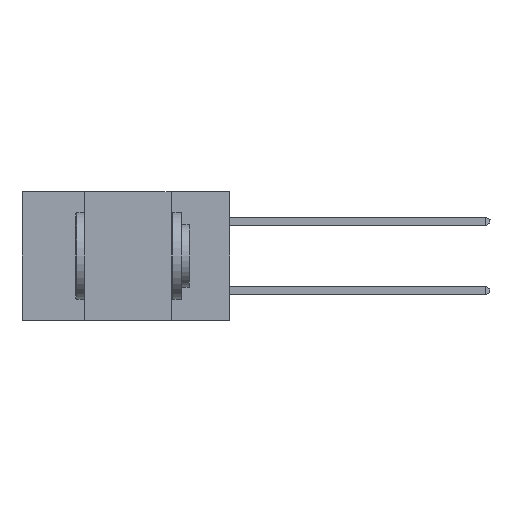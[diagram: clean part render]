
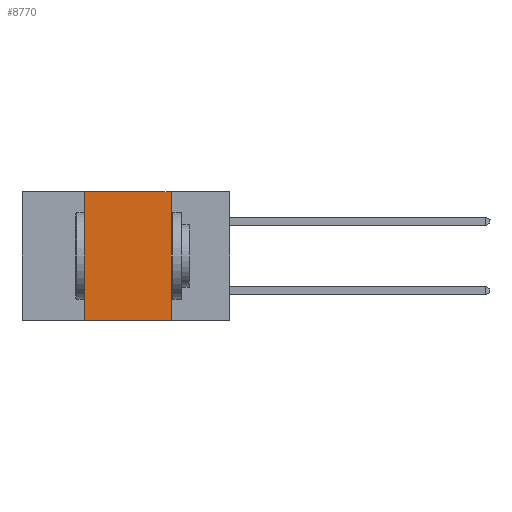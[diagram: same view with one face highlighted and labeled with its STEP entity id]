
A CAD part, left-side view. The second image highlights one B-rep face of the part: STEP entity #8770.
In plain terms, the highlighted planar face has unit normal (-1, 0, 0).
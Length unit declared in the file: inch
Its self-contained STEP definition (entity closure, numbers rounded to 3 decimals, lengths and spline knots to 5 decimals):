
#279 = LINE ( 'NONE', #2073, #4026 ) ;
#503 = VECTOR ( 'NONE', #13546, 39.37008 ) ;
#505 = ORIENTED_EDGE ( 'NONE', *, *, #21737, .F. ) ;
#1359 = ORIENTED_EDGE ( 'NONE', *, *, #23906, .F. ) ;
#1633 = CARTESIAN_POINT ( 'NONE',  ( 0., 0.42, -0.37 ) ) ;
#1995 = DIRECTION ( 'NONE',  ( 0., 0., 1. ) ) ;
#2073 = CARTESIAN_POINT ( 'NONE',  ( 0., 0.42, 0. ) ) ;
#3276 = DIRECTION ( 'NONE',  ( 0., 0., -1. ) ) ;
#4026 = VECTOR ( 'NONE', #1995, 39.37008 ) ;
#4252 = VERTEX_POINT ( 'NONE', #14264 ) ;
#5043 = CARTESIAN_POINT ( 'NONE',  ( 0., 0.6, -0.37 ) ) ;
#5609 = CARTESIAN_POINT ( 'NONE',  ( 0., 0.17, -0.37 ) ) ;
#6620 = EDGE_CURVE ( 'NONE', #19452, #16352, #10635, .T. ) ;
#7560 = ORIENTED_EDGE ( 'NONE', *, *, #20648, .F. ) ;
#8306 = ORIENTED_EDGE ( 'NONE', *, *, #6620, .T. ) ;
#8770 = ADVANCED_FACE ( 'NONE', ( #14324 ), #23129, .F. ) ;
#9388 = VERTEX_POINT ( 'NONE', #19105 ) ;
#10635 = LINE ( 'NONE', #5043, #19389 ) ;
#11601 = VECTOR ( 'NONE', #3276, 39.37008 ) ;
#11849 = CARTESIAN_POINT ( 'NONE',  ( 0., 0.6, 0. ) ) ;
#13176 = LINE ( 'NONE', #11849, #503 ) ;
#13546 = DIRECTION ( 'NONE',  ( 0., -1., 0. ) ) ;
#14264 = CARTESIAN_POINT ( 'NONE',  ( 0., 0.42, 0. ) ) ;
#14324 = FACE_OUTER_BOUND ( 'NONE', #21234, .T. ) ;
#14681 = CARTESIAN_POINT ( 'NONE',  ( 0., 0.6, 0. ) ) ;
#16143 = DIRECTION ( 'NONE',  ( 0., 0., -1. ) ) ;
#16352 = VERTEX_POINT ( 'NONE', #5609 ) ;
#17718 = LINE ( 'NONE', #18416, #11601 ) ;
#18416 = CARTESIAN_POINT ( 'NONE',  ( 0., 0.17, 0. ) ) ;
#19105 = CARTESIAN_POINT ( 'NONE',  ( 0., 0.17, 0. ) ) ;
#19389 = VECTOR ( 'NONE', #20227, 39.37008 ) ;
#19452 = VERTEX_POINT ( 'NONE', #1633 ) ;
#19833 = DIRECTION ( 'NONE',  ( 1., 0., 0. ) ) ;
#20227 = DIRECTION ( 'NONE',  ( 0., -1., 0. ) ) ;
#20648 = EDGE_CURVE ( 'NONE', #19452, #4252, #279, .T. ) ;
#21234 = EDGE_LOOP ( 'NONE', ( #1359, #505, #7560, #8306 ) ) ;
#21737 = EDGE_CURVE ( 'NONE', #4252, #9388, #13176, .T. ) ;
#22809 = AXIS2_PLACEMENT_3D ( 'NONE', #14681, #19833, #16143 ) ;
#23129 = PLANE ( 'NONE',  #22809 ) ;
#23906 = EDGE_CURVE ( 'NONE', #9388, #16352, #17718, .T. ) ;
